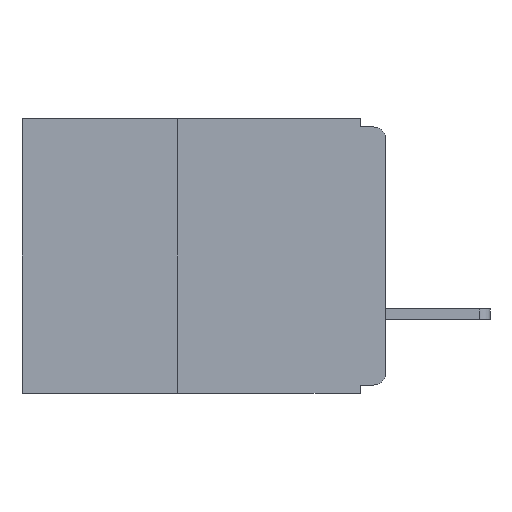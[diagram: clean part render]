
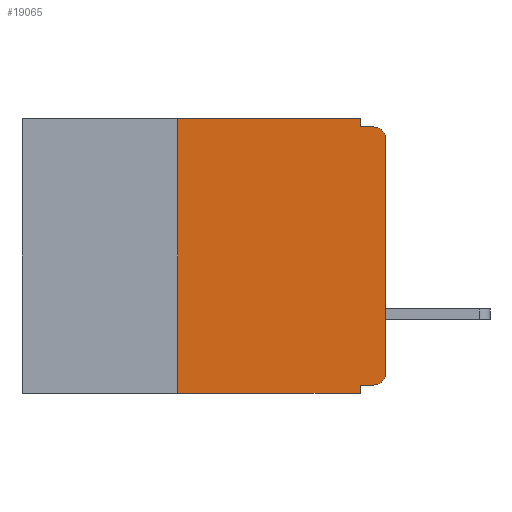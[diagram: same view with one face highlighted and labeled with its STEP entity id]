
A CAD part, left-side view. The second image highlights one B-rep face of the part: STEP entity #19065.
In plain terms, the highlighted planar face has unit normal (-1, 0, 0).
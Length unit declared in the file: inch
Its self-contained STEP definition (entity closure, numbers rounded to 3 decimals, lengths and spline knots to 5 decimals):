
#1425 = CARTESIAN_POINT ( 'NONE',  ( 0., 0., -0.305 ) ) ;
#2753 = EDGE_CURVE ( 'NONE', #27296, #11075, #15217, .T. ) ;
#3026 = EDGE_CURVE ( 'NONE', #3827, #13099, #24159, .T. ) ;
#3312 = DIRECTION ( 'NONE',  ( 0., 0., -1. ) ) ;
#3552 = CARTESIAN_POINT ( 'NONE',  ( 0., 0., -0.01 ) ) ;
#3827 = VERTEX_POINT ( 'NONE', #25576 ) ;
#4023 = VECTOR ( 'NONE', #27313, 39.37008 ) ;
#4820 = EDGE_CURVE ( 'NONE', #25037, #24333, #21195, .T. ) ;
#5478 = EDGE_LOOP ( 'NONE', ( #20035, #14884, #13357, #25296, #11706, #24923, #15103, #28747, #8521, #22339 ) ) ;
#5563 = LINE ( 'NONE', #26569, #6288 ) ;
#5870 = DIRECTION ( 'NONE',  ( 0., -1., 0. ) ) ;
#6288 = VECTOR ( 'NONE', #15177, 39.37008 ) ;
#7141 = CARTESIAN_POINT ( 'NONE',  ( 0., 0., -0.32 ) ) ;
#7520 = LINE ( 'NONE', #24163, #24977 ) ;
#8166 = VECTOR ( 'NONE', #20805, 39.37008 ) ;
#8521 = ORIENTED_EDGE ( 'NONE', *, *, #13721, .F. ) ;
#8627 = AXIS2_PLACEMENT_3D ( 'NONE', #12029, #27935, #14294 ) ;
#9522 = CIRCLE ( 'NONE', #8627, 0.015 ) ;
#9557 = CARTESIAN_POINT ( 'NONE',  ( 0., 0.031, -0.33 ) ) ;
#9827 = VECTOR ( 'NONE', #5870, 39.37008 ) ;
#10183 = LINE ( 'NONE', #25052, #4023 ) ;
#10536 = DIRECTION ( 'NONE',  ( -1., 0., 0. ) ) ;
#10917 = CARTESIAN_POINT ( 'NONE',  ( 0., 0.015, -0.32 ) ) ;
#11075 = VERTEX_POINT ( 'NONE', #13819 ) ;
#11231 = EDGE_CURVE ( 'NONE', #21943, #14944, #9522, .T. ) ;
#11706 = ORIENTED_EDGE ( 'NONE', *, *, #20312, .F. ) ;
#12029 = CARTESIAN_POINT ( 'NONE',  ( 0., 0.015, -0.305 ) ) ;
#12156 = CARTESIAN_POINT ( 'NONE',  ( 0., 0.031, -0.33 ) ) ;
#12246 = EDGE_CURVE ( 'NONE', #24333, #22898, #27986, .T. ) ;
#12356 = DIRECTION ( 'NONE',  ( 0., 0., -1. ) ) ;
#12787 = DIRECTION ( 'NONE',  ( 0., -1., 0. ) ) ;
#13099 = VERTEX_POINT ( 'NONE', #9557 ) ;
#13357 = ORIENTED_EDGE ( 'NONE', *, *, #12246, .F. ) ;
#13721 = EDGE_CURVE ( 'NONE', #21943, #3827, #14903, .T. ) ;
#13819 = CARTESIAN_POINT ( 'NONE',  ( 0., 0.25, 0. ) ) ;
#13983 = EDGE_CURVE ( 'NONE', #17824, #22898, #25979, .T. ) ;
#14036 = EDGE_CURVE ( 'NONE', #14944, #17824, #5563, .T. ) ;
#14294 = DIRECTION ( 'NONE',  ( 0., 0., -1. ) ) ;
#14513 = VECTOR ( 'NONE', #20171, 39.37008 ) ;
#14744 = CARTESIAN_POINT ( 'NONE',  ( 0., 0.437, 0. ) ) ;
#14884 = ORIENTED_EDGE ( 'NONE', *, *, #13983, .T. ) ;
#14903 = LINE ( 'NONE', #7141, #8166 ) ;
#14944 = VERTEX_POINT ( 'NONE', #1425 ) ;
#15079 = VECTOR ( 'NONE', #28935, 39.37008 ) ;
#15103 = ORIENTED_EDGE ( 'NONE', *, *, #23900, .T. ) ;
#15177 = DIRECTION ( 'NONE',  ( 0., 0., 1. ) ) ;
#15217 = LINE ( 'NONE', #19819, #14513 ) ;
#16018 = FACE_OUTER_BOUND ( 'NONE', #5478, .T. ) ;
#16702 = AXIS2_PLACEMENT_3D ( 'NONE', #24190, #10536, #26472 ) ;
#17035 = DIRECTION ( 'NONE',  ( 1., 0., 0. ) ) ;
#17824 = VERTEX_POINT ( 'NONE', #23413 ) ;
#19065 = ADVANCED_FACE ( 'NONE', ( #16018 ), #28387, .F. ) ;
#19819 = CARTESIAN_POINT ( 'NONE',  ( 0., 0.25, -0.33 ) ) ;
#20035 = ORIENTED_EDGE ( 'NONE', *, *, #14036, .T. ) ;
#20171 = DIRECTION ( 'NONE',  ( 0., 0., 1. ) ) ;
#20291 = AXIS2_PLACEMENT_3D ( 'NONE', #14744, #17035, #3312 ) ;
#20312 = EDGE_CURVE ( 'NONE', #11075, #25037, #10183, .T. ) ;
#20805 = DIRECTION ( 'NONE',  ( 0., 1., 0. ) ) ;
#21195 = LINE ( 'NONE', #29305, #15079 ) ;
#21244 = CARTESIAN_POINT ( 'NONE',  ( 0., 0.015, -0.01 ) ) ;
#21943 = VERTEX_POINT ( 'NONE', #10917 ) ;
#22339 = ORIENTED_EDGE ( 'NONE', *, *, #11231, .T. ) ;
#22898 = VERTEX_POINT ( 'NONE', #21244 ) ;
#23413 = CARTESIAN_POINT ( 'NONE',  ( 0., 0., -0.025 ) ) ;
#23448 = VECTOR ( 'NONE', #12356, 39.37008 ) ;
#23900 = EDGE_CURVE ( 'NONE', #27296, #13099, #7520, .T. ) ;
#24159 = LINE ( 'NONE', #12156, #23448 ) ;
#24163 = CARTESIAN_POINT ( 'NONE',  ( 0., 0.437, -0.33 ) ) ;
#24190 = CARTESIAN_POINT ( 'NONE',  ( 0., 0.015, -0.025 ) ) ;
#24333 = VERTEX_POINT ( 'NONE', #29633 ) ;
#24347 = CARTESIAN_POINT ( 'NONE',  ( 0., 0.25, -0.33 ) ) ;
#24923 = ORIENTED_EDGE ( 'NONE', *, *, #2753, .F. ) ;
#24977 = VECTOR ( 'NONE', #12787, 39.37008 ) ;
#25037 = VERTEX_POINT ( 'NONE', #27606 ) ;
#25052 = CARTESIAN_POINT ( 'NONE',  ( 0., 0.437, 0. ) ) ;
#25296 = ORIENTED_EDGE ( 'NONE', *, *, #4820, .F. ) ;
#25576 = CARTESIAN_POINT ( 'NONE',  ( 0., 0.031, -0.32 ) ) ;
#25979 = CIRCLE ( 'NONE', #16702, 0.015 ) ;
#26472 = DIRECTION ( 'NONE',  ( 0., 0., -1. ) ) ;
#26569 = CARTESIAN_POINT ( 'NONE',  ( 0., 0., 0. ) ) ;
#27296 = VERTEX_POINT ( 'NONE', #24347 ) ;
#27313 = DIRECTION ( 'NONE',  ( 0., -1., 0. ) ) ;
#27606 = CARTESIAN_POINT ( 'NONE',  ( 0., 0.031, 0. ) ) ;
#27935 = DIRECTION ( 'NONE',  ( -1., 0., 0. ) ) ;
#27986 = LINE ( 'NONE', #3552, #9827 ) ;
#28387 = PLANE ( 'NONE',  #20291 ) ;
#28747 = ORIENTED_EDGE ( 'NONE', *, *, #3026, .F. ) ;
#28935 = DIRECTION ( 'NONE',  ( 0., 0., -1. ) ) ;
#29305 = CARTESIAN_POINT ( 'NONE',  ( 0., 0.031, 0. ) ) ;
#29633 = CARTESIAN_POINT ( 'NONE',  ( 0., 0.031, -0.01 ) ) ;
